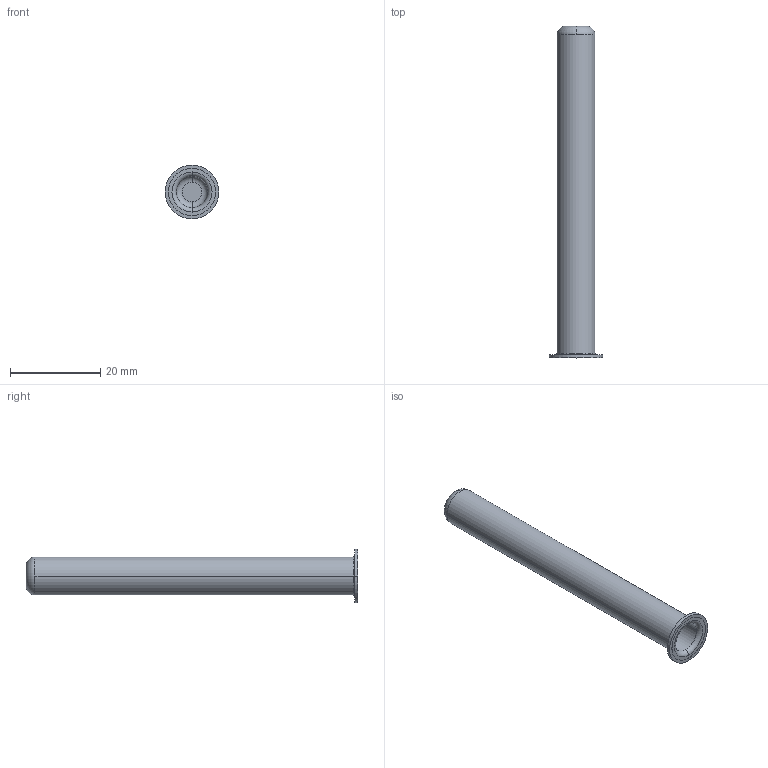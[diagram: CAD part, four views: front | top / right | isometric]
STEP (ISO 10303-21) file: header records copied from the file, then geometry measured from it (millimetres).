
FILE_DESCRIPTION (( 'STEP AP214' ), '1' );
FILE_NAME ('Recoil Spring Guide.step', '2014-07-30T19:46:38', ( 'WarFairy' ), ( '' ), 'SwSTEP 2.0', 'SolidWorks 2013', '' );
FILE_SCHEMA (( 'AUTOMOTIVE_DESIGN' ));
Length unit declared in the file: millimetre
Products named in the file (1): Recoil Spring Guide
Bounding box: 11.9 x 73.48 x 11.9 mm (x, y, z)
Volume: 1309.3 mm3; surface area: 3708.6 mm2
Topology: 1 solids, 1 shells, 21 faces, 48 edges, 32 vertices
Faces by surface type: torus 8, cylinder 8, plane 5
Entity records: 656 total; most frequent: DIRECTION 132, CARTESIAN_POINT 102, ORIENTED_EDGE 96, AXIS2_PLACEMENT_3D 62, EDGE_CURVE 48, CIRCLE 40, VERTEX_POINT 32, EDGE_LOOP 24
